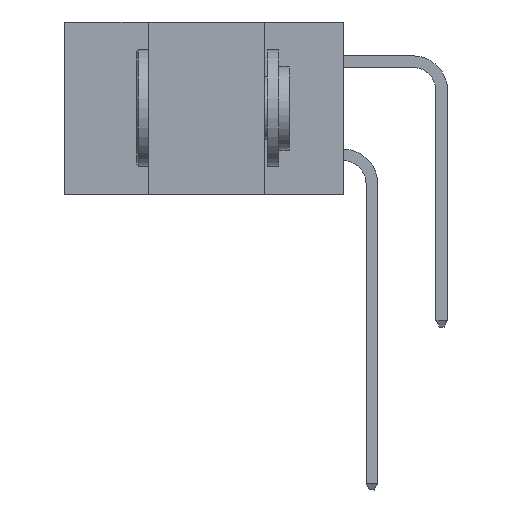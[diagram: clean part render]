
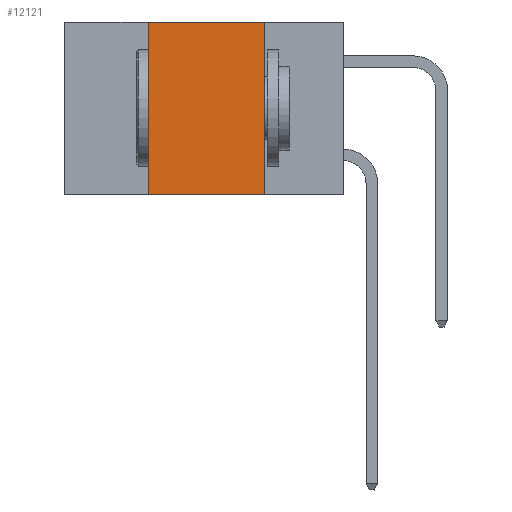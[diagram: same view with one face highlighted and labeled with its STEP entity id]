
A CAD part, left-side view. The second image highlights one B-rep face of the part: STEP entity #12121.
In plain terms, the highlighted planar face has unit normal (-1, 0, 0).
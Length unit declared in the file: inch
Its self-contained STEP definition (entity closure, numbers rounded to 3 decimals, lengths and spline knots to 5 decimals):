
#428 = LINE ( 'NONE', #17014, #7262 ) ;
#582 = LINE ( 'NONE', #3374, #6335 ) ;
#923 = EDGE_CURVE ( 'NONE', #15198, #12076, #17593, .T. ) ;
#1221 = CARTESIAN_POINT ( 'NONE',  ( 0., 0.42, -0.37 ) ) ;
#2273 = DIRECTION ( 'NONE',  ( 0., 0., -1. ) ) ;
#3334 = ORIENTED_EDGE ( 'NONE', *, *, #7593, .T. ) ;
#3374 = CARTESIAN_POINT ( 'NONE',  ( 0., 0.6, 0. ) ) ;
#3542 = ORIENTED_EDGE ( 'NONE', *, *, #923, .F. ) ;
#3624 = CARTESIAN_POINT ( 'NONE',  ( 0., 0.42, -0.37 ) ) ;
#3741 = CARTESIAN_POINT ( 'NONE',  ( 0., 0.17, 0. ) ) ;
#4030 = CARTESIAN_POINT ( 'NONE',  ( 0., 0.17, -0.37 ) ) ;
#4122 = PLANE ( 'NONE',  #16375 ) ;
#4184 = VECTOR ( 'NONE', #13084, 39.37008 ) ;
#5492 = CARTESIAN_POINT ( 'NONE',  ( 0., 0.6, 0. ) ) ;
#6072 = CARTESIAN_POINT ( 'NONE',  ( 0., 0.42, 0. ) ) ;
#6221 = LINE ( 'NONE', #8936, #4184 ) ;
#6335 = VECTOR ( 'NONE', #7625, 39.37008 ) ;
#7262 = VECTOR ( 'NONE', #12885, 39.37008 ) ;
#7593 = EDGE_CURVE ( 'NONE', #15198, #9801, #428, .T. ) ;
#7625 = DIRECTION ( 'NONE',  ( 0., -1., 0. ) ) ;
#7872 = FACE_OUTER_BOUND ( 'NONE', #13534, .T. ) ;
#7874 = DIRECTION ( 'NONE',  ( 0., 0., 1. ) ) ;
#8936 = CARTESIAN_POINT ( 'NONE',  ( 0., 0.17, -0.37 ) ) ;
#9801 = VERTEX_POINT ( 'NONE', #4030 ) ;
#10145 = ORIENTED_EDGE ( 'NONE', *, *, #12888, .F. ) ;
#11144 = EDGE_CURVE ( 'NONE', #14475, #9801, #6221, .T. ) ;
#12027 = DIRECTION ( 'NONE',  ( 1., 0., 0. ) ) ;
#12076 = VERTEX_POINT ( 'NONE', #6072 ) ;
#12121 = ADVANCED_FACE ( 'NONE', ( #7872 ), #4122, .F. ) ;
#12885 = DIRECTION ( 'NONE',  ( 0., -1., 0. ) ) ;
#12888 = EDGE_CURVE ( 'NONE', #12076, #14475, #582, .T. ) ;
#13084 = DIRECTION ( 'NONE',  ( 0., 0., -1. ) ) ;
#13534 = EDGE_LOOP ( 'NONE', ( #17515, #10145, #3542, #3334 ) ) ;
#14475 = VERTEX_POINT ( 'NONE', #3741 ) ;
#15198 = VERTEX_POINT ( 'NONE', #1221 ) ;
#16375 = AXIS2_PLACEMENT_3D ( 'NONE', #5492, #12027, #2273 ) ;
#17014 = CARTESIAN_POINT ( 'NONE',  ( 0., 0.6, -0.37 ) ) ;
#17515 = ORIENTED_EDGE ( 'NONE', *, *, #11144, .F. ) ;
#17593 = LINE ( 'NONE', #3624, #17662 ) ;
#17662 = VECTOR ( 'NONE', #7874, 39.37008 ) ;
